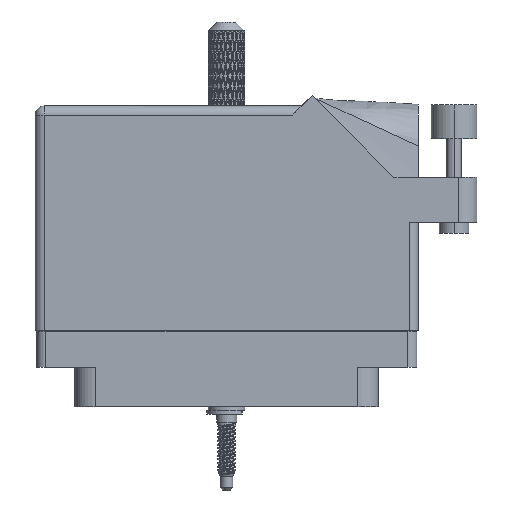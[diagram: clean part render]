
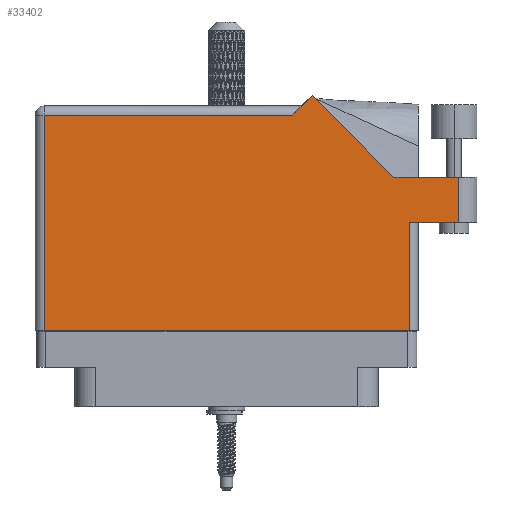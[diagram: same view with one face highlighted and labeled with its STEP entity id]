
A CAD part, front view. The second image highlights one B-rep face of the part: STEP entity #33402.
In plain terms, the highlighted face is planar.
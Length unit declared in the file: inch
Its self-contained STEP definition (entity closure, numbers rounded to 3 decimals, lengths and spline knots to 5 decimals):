
#2379 = CARTESIAN_POINT ( 'NONE',  ( -1.244, -0.1, 0.455 ) ) ;
#3420 = VECTOR ( 'NONE', #90757, 39.37008 ) ;
#8338 = ORIENTED_EDGE ( 'NONE', *, *, #43273, .T. ) ;
#10901 = VECTOR ( 'NONE', #100778, 39.37008 ) ;
#13831 = VERTEX_POINT ( 'NONE', #84023 ) ;
#14970 = DIRECTION ( 'NONE',  ( -0.707, -0.707, 0. ) ) ;
#15568 = CARTESIAN_POINT ( 'NONE',  ( 0.513, 1.43, 0.455 ) ) ;
#17217 = ORIENTED_EDGE ( 'NONE', *, *, #96250, .T. ) ;
#21411 = CARTESIAN_POINT ( 'NONE',  ( 1.244, 0.637, 0.455 ) ) ;
#22361 = DIRECTION ( 'NONE',  ( 0., 1., 0. ) ) ;
#24215 = ORIENTED_EDGE ( 'NONE', *, *, #80917, .T. ) ;
#27536 = VECTOR ( 'NONE', #22361, 39.37008 ) ;
#29192 = CARTESIAN_POINT ( 'NONE',  ( 0.58371, 1.50071, 0.455 ) ) ;
#30362 = LINE ( 'NONE', #57735, #91556 ) ;
#32952 = VECTOR ( 'NONE', #85546, 39.37008 ) ;
#33402 = ADVANCED_FACE ( 'NONE', ( #50486 ), #105771, .F. ) ;
#36229 = ORIENTED_EDGE ( 'NONE', *, *, #93154, .T. ) ;
#36584 = LINE ( 'NONE', #46691, #3420 ) ;
#39117 = LINE ( 'NONE', #112301, #32952 ) ;
#40141 = VERTEX_POINT ( 'NONE', #2379 ) ;
#40963 = CARTESIAN_POINT ( 'NONE',  ( -1.306, 1.43, 0.455 ) ) ;
#43273 = EDGE_CURVE ( 'NONE', #94593, #40141, #108542, .T. ) ;
#45044 = CARTESIAN_POINT ( 'NONE',  ( 1.581, 0.637, 0.455 ) ) ;
#45706 = CARTESIAN_POINT ( 'NONE',  ( -1.306, -0.1, 0.455 ) ) ;
#46284 = DIRECTION ( 'NONE',  ( 1., 0., 0. ) ) ;
#46691 = CARTESIAN_POINT ( 'NONE',  ( -1.306, 1.368, 0.455 ) ) ;
#50303 = AXIS2_PLACEMENT_3D ( 'NONE', #40963, #115314, #58821 ) ;
#50486 = FACE_OUTER_BOUND ( 'NONE', #55478, .T. ) ;
#50907 = LINE ( 'NONE', #96711, #27536 ) ;
#53291 = EDGE_CURVE ( 'NONE', #40141, #13831, #92673, .T. ) ;
#53735 = VERTEX_POINT ( 'NONE', #106141 ) ;
#53805 = CARTESIAN_POINT ( 'NONE',  ( -1.244, -0.1, 0.455 ) ) ;
#55183 = VERTEX_POINT ( 'NONE', #45044 ) ;
#55478 = EDGE_LOOP ( 'NONE', ( #24215, #36229, #94627, #104526, #17217, #113786, #8338, #98982, #86056 ) ) ;
#56469 = VECTOR ( 'NONE', #113592, 39.37008 ) ;
#57735 = CARTESIAN_POINT ( 'NONE',  ( 1.581, 0.944, 0.455 ) ) ;
#58260 = CARTESIAN_POINT ( 'NONE',  ( 1.306, 0.637, 0.455 ) ) ;
#58328 = EDGE_CURVE ( 'NONE', #13831, #73261, #50907, .T. ) ;
#58821 = DIRECTION ( 'NONE',  ( -1., 0., 0. ) ) ;
#69210 = CARTESIAN_POINT ( 'NONE',  ( 0.451, 1.368, 0.455 ) ) ;
#71673 = EDGE_CURVE ( 'NONE', #92010, #94593, #36584, .T. ) ;
#71814 = CARTESIAN_POINT ( 'NONE',  ( -1.244, 1.368, 0.455 ) ) ;
#73261 = VERTEX_POINT ( 'NONE', #21411 ) ;
#73510 = VERTEX_POINT ( 'NONE', #29192 ) ;
#74051 = VECTOR ( 'NONE', #105947, 39.37008 ) ;
#74730 = VECTOR ( 'NONE', #14970, 39.37008 ) ;
#75325 = EDGE_CURVE ( 'NONE', #53735, #103219, #89288, .T. ) ;
#80917 = EDGE_CURVE ( 'NONE', #73261, #55183, #111803, .T. ) ;
#84023 = CARTESIAN_POINT ( 'NONE',  ( 1.244, -0.1, 0.455 ) ) ;
#85546 = DIRECTION ( 'NONE',  ( -0.707, 0.707, 0. ) ) ;
#86056 = ORIENTED_EDGE ( 'NONE', *, *, #58328, .T. ) ;
#89288 = LINE ( 'NONE', #114906, #74051 ) ;
#90757 = DIRECTION ( 'NONE',  ( -1., 0., 0. ) ) ;
#91556 = VECTOR ( 'NONE', #94039, 39.37008 ) ;
#92010 = VERTEX_POINT ( 'NONE', #69210 ) ;
#92200 = CARTESIAN_POINT ( 'NONE',  ( 1.14042, 0.944, 0.455 ) ) ;
#92673 = LINE ( 'NONE', #45706, #101153 ) ;
#93154 = EDGE_CURVE ( 'NONE', #55183, #53735, #30362, .T. ) ;
#94039 = DIRECTION ( 'NONE',  ( 0., 1., 0. ) ) ;
#94593 = VERTEX_POINT ( 'NONE', #71814 ) ;
#94627 = ORIENTED_EDGE ( 'NONE', *, *, #75325, .T. ) ;
#95925 = EDGE_CURVE ( 'NONE', #103219, #73510, #39117, .T. ) ;
#96250 = EDGE_CURVE ( 'NONE', #73510, #92010, #96511, .T. ) ;
#96511 = LINE ( 'NONE', #15568, #74730 ) ;
#96711 = CARTESIAN_POINT ( 'NONE',  ( 1.244, 0.637, 0.455 ) ) ;
#98982 = ORIENTED_EDGE ( 'NONE', *, *, #53291, .T. ) ;
#100778 = DIRECTION ( 'NONE',  ( 0., -1., 0. ) ) ;
#101153 = VECTOR ( 'NONE', #46284, 39.37008 ) ;
#103219 = VERTEX_POINT ( 'NONE', #92200 ) ;
#104526 = ORIENTED_EDGE ( 'NONE', *, *, #95925, .T. ) ;
#105771 = PLANE ( 'NONE',  #50303 ) ;
#105947 = DIRECTION ( 'NONE',  ( -1., 0., 0. ) ) ;
#106141 = CARTESIAN_POINT ( 'NONE',  ( 1.581, 0.944, 0.455 ) ) ;
#108542 = LINE ( 'NONE', #53805, #10901 ) ;
#111803 = LINE ( 'NONE', #58260, #56469 ) ;
#112301 = CARTESIAN_POINT ( 'NONE',  ( 1.14042, 0.944, 0.455 ) ) ;
#113592 = DIRECTION ( 'NONE',  ( 1., 0., 0. ) ) ;
#113786 = ORIENTED_EDGE ( 'NONE', *, *, #71673, .T. ) ;
#114906 = CARTESIAN_POINT ( 'NONE',  ( 1.706, 0.944, 0.455 ) ) ;
#115314 = DIRECTION ( 'NONE',  ( 0., 0., -1. ) ) ;
